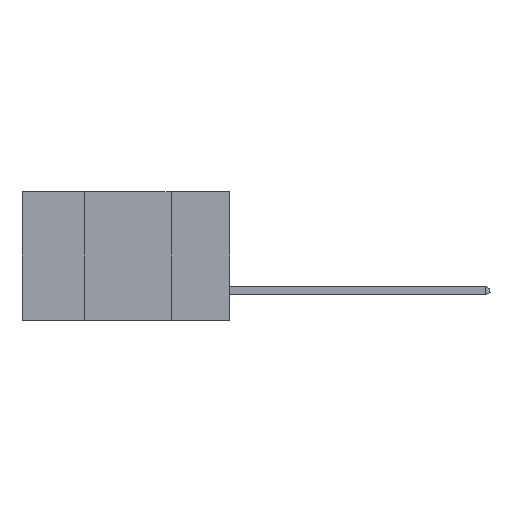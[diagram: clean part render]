
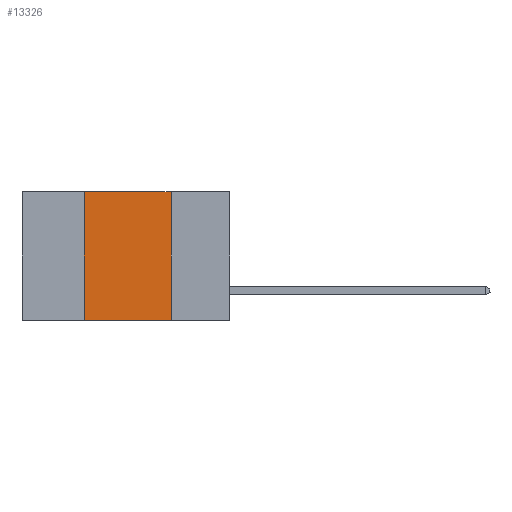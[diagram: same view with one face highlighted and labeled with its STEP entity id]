
A CAD part, left-side view. The second image highlights one B-rep face of the part: STEP entity #13326.
In plain terms, the highlighted planar face has unit normal (-1, 0, 0).
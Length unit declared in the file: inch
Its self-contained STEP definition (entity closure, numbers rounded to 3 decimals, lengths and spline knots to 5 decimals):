
#275 = ORIENTED_EDGE ( 'NONE', *, *, #23857, .F. ) ;
#2472 = DIRECTION ( 'NONE',  ( 0., 0., -1. ) ) ;
#4614 = CARTESIAN_POINT ( 'NONE',  ( 0., 0.42, -0.37 ) ) ;
#6444 = VERTEX_POINT ( 'NONE', #13229 ) ;
#6778 = LINE ( 'NONE', #24751, #29368 ) ;
#8018 = CARTESIAN_POINT ( 'NONE',  ( 0., 0.17, -0.37 ) ) ;
#8293 = ORIENTED_EDGE ( 'NONE', *, *, #29166, .T. ) ;
#8412 = VECTOR ( 'NONE', #25435, 39.37008 ) ;
#10396 = DIRECTION ( 'NONE',  ( 0., -1., 0. ) ) ;
#10872 = DIRECTION ( 'NONE',  ( 0., 0., -1. ) ) ;
#11465 = LINE ( 'NONE', #20173, #15203 ) ;
#11599 = LINE ( 'NONE', #29240, #16842 ) ;
#11931 = DIRECTION ( 'NONE',  ( 1., 0., 0. ) ) ;
#13229 = CARTESIAN_POINT ( 'NONE',  ( 0., 0.42, 0. ) ) ;
#13326 = ADVANCED_FACE ( 'NONE', ( #28411 ), #21180, .F. ) ;
#14061 = CARTESIAN_POINT ( 'NONE',  ( 0., 0.42, 0. ) ) ;
#15203 = VECTOR ( 'NONE', #10396, 39.37008 ) ;
#15225 = VERTEX_POINT ( 'NONE', #4614 ) ;
#16842 = VECTOR ( 'NONE', #17453, 39.37008 ) ;
#17453 = DIRECTION ( 'NONE',  ( 0., -1., 0. ) ) ;
#18912 = CARTESIAN_POINT ( 'NONE',  ( 0., 0.6, 0. ) ) ;
#19371 = VERTEX_POINT ( 'NONE', #8018 ) ;
#19703 = CARTESIAN_POINT ( 'NONE',  ( 0., 0.17, 0. ) ) ;
#19964 = AXIS2_PLACEMENT_3D ( 'NONE', #18912, #11931, #2472 ) ;
#20173 = CARTESIAN_POINT ( 'NONE',  ( 0., 0.6, 0. ) ) ;
#21180 = PLANE ( 'NONE',  #19964 ) ;
#21479 = VERTEX_POINT ( 'NONE', #19703 ) ;
#22370 = EDGE_CURVE ( 'NONE', #21479, #19371, #6778, .T. ) ;
#22995 = EDGE_LOOP ( 'NONE', ( #27088, #275, #27742, #8293 ) ) ;
#23857 = EDGE_CURVE ( 'NONE', #6444, #21479, #11465, .T. ) ;
#24751 = CARTESIAN_POINT ( 'NONE',  ( 0., 0.17, 0. ) ) ;
#25435 = DIRECTION ( 'NONE',  ( 0., 0., 1. ) ) ;
#25914 = EDGE_CURVE ( 'NONE', #15225, #6444, #27290, .T. ) ;
#27088 = ORIENTED_EDGE ( 'NONE', *, *, #22370, .F. ) ;
#27290 = LINE ( 'NONE', #14061, #8412 ) ;
#27742 = ORIENTED_EDGE ( 'NONE', *, *, #25914, .F. ) ;
#28411 = FACE_OUTER_BOUND ( 'NONE', #22995, .T. ) ;
#29166 = EDGE_CURVE ( 'NONE', #15225, #19371, #11599, .T. ) ;
#29240 = CARTESIAN_POINT ( 'NONE',  ( 0., 0.6, -0.37 ) ) ;
#29368 = VECTOR ( 'NONE', #10872, 39.37008 ) ;
